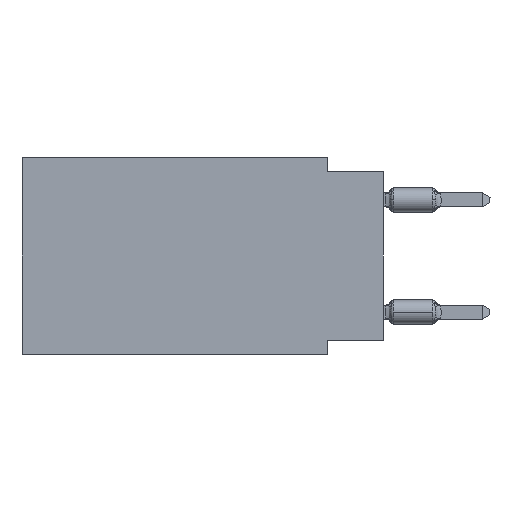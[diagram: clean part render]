
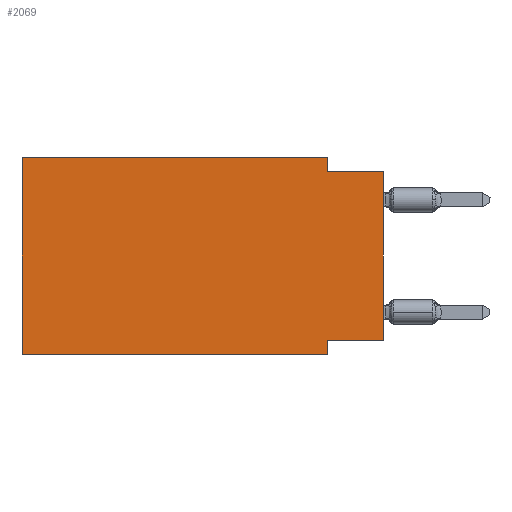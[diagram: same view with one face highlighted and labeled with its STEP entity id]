
A CAD part, left-side view. The second image highlights one B-rep face of the part: STEP entity #2069.
In plain terms, the highlighted planar face has unit normal (-1, 0, 0).
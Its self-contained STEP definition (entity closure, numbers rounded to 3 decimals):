
#44 = ORIENTED_EDGE ( 'NONE', *, *, #52435, .F. ) ;
#1284 = FACE_OUTER_BOUND ( 'NONE', #54186, .T. ) ;
#2069 = ADVANCED_FACE ( 'NONE', ( #1284 ), #29430, .F. ) ;
#2948 = LINE ( 'NONE', #36237, #51552 ) ;
#3445 = DIRECTION ( 'NONE',  ( 0., 0., -1. ) ) ;
#3829 = DIRECTION ( 'NONE',  ( 0., 0., 1. ) ) ;
#4483 = CARTESIAN_POINT ( 'NONE',  ( 0., 2.54, -8.89 ) ) ;
#5355 = EDGE_CURVE ( 'NONE', #11871, #16847, #9008, .T. ) ;
#6101 = DIRECTION ( 'NONE',  ( 0., 0., -1. ) ) ;
#6672 = VECTOR ( 'NONE', #25978, 1000. ) ;
#7500 = LINE ( 'NONE', #24795, #6672 ) ;
#7602 = ORIENTED_EDGE ( 'NONE', *, *, #51289, .T. ) ;
#7986 = VECTOR ( 'NONE', #46534, 1000. ) ;
#9008 = LINE ( 'NONE', #56270, #7986 ) ;
#9092 = VERTEX_POINT ( 'NONE', #39374 ) ;
#11538 = VERTEX_POINT ( 'NONE', #55690 ) ;
#11871 = VERTEX_POINT ( 'NONE', #19250 ) ;
#12404 = ORIENTED_EDGE ( 'NONE', *, *, #5355, .F. ) ;
#12954 = VECTOR ( 'NONE', #29314, 1000. ) ;
#13423 = LINE ( 'NONE', #21908, #43521 ) ;
#13881 = ORIENTED_EDGE ( 'NONE', *, *, #16197, .T. ) ;
#15383 = LINE ( 'NONE', #16275, #12954 ) ;
#15478 = VERTEX_POINT ( 'NONE', #26907 ) ;
#15861 = VECTOR ( 'NONE', #26345, 1000. ) ;
#16197 = EDGE_CURVE ( 'NONE', #11538, #16847, #24099, .T. ) ;
#16275 = CARTESIAN_POINT ( 'NONE',  ( 0., 16.383, 0. ) ) ;
#16847 = VERTEX_POINT ( 'NONE', #4483 ) ;
#19250 = CARTESIAN_POINT ( 'NONE',  ( 0., 2.54, -8.255 ) ) ;
#20634 = CARTESIAN_POINT ( 'NONE',  ( 0., 16.383, 0. ) ) ;
#21787 = CARTESIAN_POINT ( 'NONE',  ( 0., 0., -0.635 ) ) ;
#21908 = CARTESIAN_POINT ( 'NONE',  ( 0., 2.54, 0. ) ) ;
#24099 = LINE ( 'NONE', #43451, #36663 ) ;
#24795 = CARTESIAN_POINT ( 'NONE',  ( 0., 0., -8.255 ) ) ;
#25978 = DIRECTION ( 'NONE',  ( 0., 1., 0. ) ) ;
#26345 = DIRECTION ( 'NONE',  ( 0., -1., 0. ) ) ;
#26907 = CARTESIAN_POINT ( 'NONE',  ( 0., 0., -0.635 ) ) ;
#27311 = VECTOR ( 'NONE', #38636, 1000. ) ;
#27490 = VERTEX_POINT ( 'NONE', #59314 ) ;
#29314 = DIRECTION ( 'NONE',  ( 0., 0., 1. ) ) ;
#29427 = ORIENTED_EDGE ( 'NONE', *, *, #47650, .F. ) ;
#29430 = PLANE ( 'NONE',  #56092 ) ;
#29894 = ORIENTED_EDGE ( 'NONE', *, *, #34965, .F. ) ;
#30119 = VERTEX_POINT ( 'NONE', #46625 ) ;
#34965 = EDGE_CURVE ( 'NONE', #50680, #11871, #7500, .T. ) ;
#36237 = CARTESIAN_POINT ( 'NONE',  ( 0., 0., 0. ) ) ;
#36663 = VECTOR ( 'NONE', #42850, 1000. ) ;
#38636 = DIRECTION ( 'NONE',  ( 0., -1., 0. ) ) ;
#39374 = CARTESIAN_POINT ( 'NONE',  ( 0., 16.383, 0. ) ) ;
#42850 = DIRECTION ( 'NONE',  ( 0., -1., 0. ) ) ;
#43451 = CARTESIAN_POINT ( 'NONE',  ( 0., 16.383, -8.89 ) ) ;
#43521 = VECTOR ( 'NONE', #3445, 1000. ) ;
#44515 = LINE ( 'NONE', #21787, #15861 ) ;
#46534 = DIRECTION ( 'NONE',  ( 0., 0., -1. ) ) ;
#46625 = CARTESIAN_POINT ( 'NONE',  ( 0., 2.54, 0. ) ) ;
#47345 = ORIENTED_EDGE ( 'NONE', *, *, #59821, .F. ) ;
#47650 = EDGE_CURVE ( 'NONE', #30119, #27490, #13423, .T. ) ;
#50439 = EDGE_CURVE ( 'NONE', #9092, #30119, #52568, .T. ) ;
#50680 = VERTEX_POINT ( 'NONE', #53070 ) ;
#51289 = EDGE_CURVE ( 'NONE', #50680, #15478, #2948, .T. ) ;
#51552 = VECTOR ( 'NONE', #3829, 1000. ) ;
#52435 = EDGE_CURVE ( 'NONE', #27490, #15478, #44515, .T. ) ;
#52568 = LINE ( 'NONE', #56840, #27311 ) ;
#53038 = ORIENTED_EDGE ( 'NONE', *, *, #50439, .F. ) ;
#53070 = CARTESIAN_POINT ( 'NONE',  ( 0., 0., -8.255 ) ) ;
#54186 = EDGE_LOOP ( 'NONE', ( #7602, #44, #29427, #53038, #47345, #13881, #12404, #29894 ) ) ;
#55690 = CARTESIAN_POINT ( 'NONE',  ( 0., 16.383, -8.89 ) ) ;
#56092 = AXIS2_PLACEMENT_3D ( 'NONE', #20634, #57312, #6101 ) ;
#56270 = CARTESIAN_POINT ( 'NONE',  ( 0., 2.54, -8.89 ) ) ;
#56840 = CARTESIAN_POINT ( 'NONE',  ( 0., 16.383, 0. ) ) ;
#57312 = DIRECTION ( 'NONE',  ( 1., 0., 0. ) ) ;
#59314 = CARTESIAN_POINT ( 'NONE',  ( 0., 2.54, -0.635 ) ) ;
#59821 = EDGE_CURVE ( 'NONE', #11538, #9092, #15383, .T. ) ;
